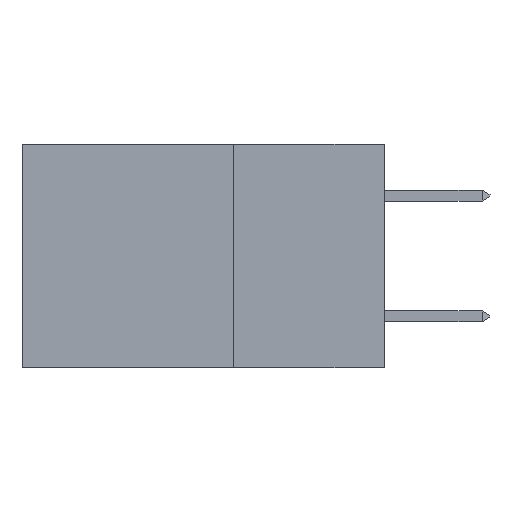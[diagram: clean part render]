
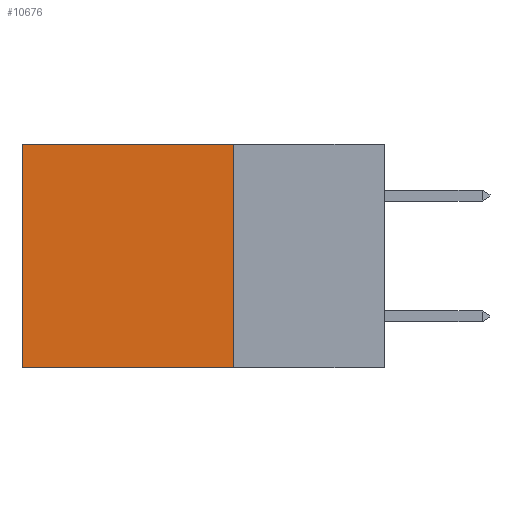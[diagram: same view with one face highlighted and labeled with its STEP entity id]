
A CAD part, left-side view. The second image highlights one B-rep face of the part: STEP entity #10676.
In plain terms, the highlighted planar face has unit normal (-1, 0, 0).
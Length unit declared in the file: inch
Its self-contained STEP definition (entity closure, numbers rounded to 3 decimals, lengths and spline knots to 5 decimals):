
#36 = CARTESIAN_POINT ( 'NONE',  ( 0.2875, 0.25, -0.37 ) ) ;
#560 = LINE ( 'NONE', #36, #2813 ) ;
#912 = CARTESIAN_POINT ( 'NONE',  ( 0.2875, 0.25, 0. ) ) ;
#1812 = CARTESIAN_POINT ( 'NONE',  ( 0.2875, 0.6, 0. ) ) ;
#1957 = DIRECTION ( 'NONE',  ( 0., 0., -1. ) ) ;
#1995 = CARTESIAN_POINT ( 'NONE',  ( 0.2875, 0.25, 0. ) ) ;
#2285 = DIRECTION ( 'NONE',  ( 0., 0., -1. ) ) ;
#2369 = CARTESIAN_POINT ( 'NONE',  ( 0.2875, 0.25, -0.37 ) ) ;
#2498 = VECTOR ( 'NONE', #1957, 39.37008 ) ;
#2813 = VECTOR ( 'NONE', #6005, 39.37008 ) ;
#2823 = ORIENTED_EDGE ( 'NONE', *, *, #10447, .T. ) ;
#3162 = DIRECTION ( 'NONE',  ( 1., 0., 0. ) ) ;
#3506 = LINE ( 'NONE', #912, #6072 ) ;
#3564 = CARTESIAN_POINT ( 'NONE',  ( 0.2875, 0.6, -0.37 ) ) ;
#3813 = CARTESIAN_POINT ( 'NONE',  ( 0.2875, 0.25, 0. ) ) ;
#4056 = VERTEX_POINT ( 'NONE', #3564 ) ;
#4212 = FACE_OUTER_BOUND ( 'NONE', #10859, .T. ) ;
#4278 = VERTEX_POINT ( 'NONE', #1812 ) ;
#4350 = LINE ( 'NONE', #6939, #2498 ) ;
#4590 = PLANE ( 'NONE',  #6455 ) ;
#4846 = DIRECTION ( 'NONE',  ( 0., 0., -1. ) ) ;
#5409 = ORIENTED_EDGE ( 'NONE', *, *, #7036, .F. ) ;
#5418 = VERTEX_POINT ( 'NONE', #2369 ) ;
#5849 = ORIENTED_EDGE ( 'NONE', *, *, #7375, .T. ) ;
#6005 = DIRECTION ( 'NONE',  ( 0., 1., 0. ) ) ;
#6072 = VECTOR ( 'NONE', #6866, 39.37008 ) ;
#6455 = AXIS2_PLACEMENT_3D ( 'NONE', #7202, #3162, #4846 ) ;
#6866 = DIRECTION ( 'NONE',  ( 0., 1., 0. ) ) ;
#6939 = CARTESIAN_POINT ( 'NONE',  ( 0.2875, 0.6, 0. ) ) ;
#7036 = EDGE_CURVE ( 'NONE', #10549, #5418, #9896, .T. ) ;
#7202 = CARTESIAN_POINT ( 'NONE',  ( 0.2875, 0.25, 0. ) ) ;
#7357 = ORIENTED_EDGE ( 'NONE', *, *, #8684, .F. ) ;
#7375 = EDGE_CURVE ( 'NONE', #10549, #4278, #3506, .T. ) ;
#8572 = VECTOR ( 'NONE', #2285, 39.37008 ) ;
#8684 = EDGE_CURVE ( 'NONE', #5418, #4056, #560, .T. ) ;
#9896 = LINE ( 'NONE', #1995, #8572 ) ;
#10447 = EDGE_CURVE ( 'NONE', #4278, #4056, #4350, .T. ) ;
#10549 = VERTEX_POINT ( 'NONE', #3813 ) ;
#10676 = ADVANCED_FACE ( 'NONE', ( #4212 ), #4590, .F. ) ;
#10859 = EDGE_LOOP ( 'NONE', ( #2823, #7357, #5409, #5849 ) ) ;
